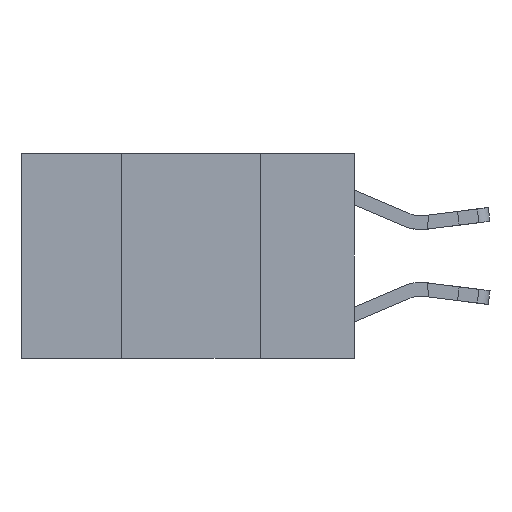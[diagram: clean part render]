
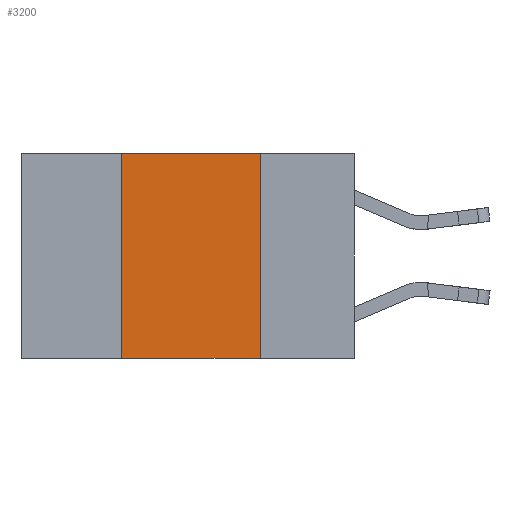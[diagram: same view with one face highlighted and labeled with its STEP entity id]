
A CAD part, left-side view. The second image highlights one B-rep face of the part: STEP entity #3200.
In plain terms, the highlighted planar face has unit normal (-1, 0, 0).
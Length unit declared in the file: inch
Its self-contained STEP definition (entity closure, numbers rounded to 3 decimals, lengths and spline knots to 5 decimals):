
#799 = VECTOR ( 'NONE', #19173, 39.37008 ) ;
#1078 = AXIS2_PLACEMENT_3D ( 'NONE', #11572, #17243, #7800 ) ;
#2281 = DIRECTION ( 'NONE',  ( 0., 0., -1. ) ) ;
#2421 = VERTEX_POINT ( 'NONE', #9214 ) ;
#2836 = VERTEX_POINT ( 'NONE', #13251 ) ;
#3200 = ADVANCED_FACE ( 'NONE', ( #12725 ), #14143, .F. ) ;
#3769 = LINE ( 'NONE', #14783, #11675 ) ;
#3931 = CARTESIAN_POINT ( 'NONE',  ( 0., 0.6, -0.37 ) ) ;
#4461 = LINE ( 'NONE', #11296, #799 ) ;
#6313 = ORIENTED_EDGE ( 'NONE', *, *, #10711, .F. ) ;
#7290 = ORIENTED_EDGE ( 'NONE', *, *, #11797, .T. ) ;
#7346 = VECTOR ( 'NONE', #13872, 39.37008 ) ;
#7543 = VERTEX_POINT ( 'NONE', #14776 ) ;
#7742 = VERTEX_POINT ( 'NONE', #16450 ) ;
#7800 = DIRECTION ( 'NONE',  ( 0., 0., -1. ) ) ;
#9214 = CARTESIAN_POINT ( 'NONE',  ( 0., 0.17, 0. ) ) ;
#10711 = EDGE_CURVE ( 'NONE', #7742, #7543, #15244, .T. ) ;
#11296 = CARTESIAN_POINT ( 'NONE',  ( 0., 0.6, 0. ) ) ;
#11572 = CARTESIAN_POINT ( 'NONE',  ( 0., 0.6, 0. ) ) ;
#11675 = VECTOR ( 'NONE', #2281, 39.37008 ) ;
#11797 = EDGE_CURVE ( 'NONE', #7742, #2836, #20089, .T. ) ;
#12265 = VECTOR ( 'NONE', #13404, 39.37008 ) ;
#12505 = EDGE_LOOP ( 'NONE', ( #15885, #12742, #6313, #7290 ) ) ;
#12725 = FACE_OUTER_BOUND ( 'NONE', #12505, .T. ) ;
#12742 = ORIENTED_EDGE ( 'NONE', *, *, #15253, .F. ) ;
#13251 = CARTESIAN_POINT ( 'NONE',  ( 0., 0.17, -0.37 ) ) ;
#13404 = DIRECTION ( 'NONE',  ( 0., -1., 0. ) ) ;
#13872 = DIRECTION ( 'NONE',  ( 0., 0., 1. ) ) ;
#13922 = EDGE_CURVE ( 'NONE', #2421, #2836, #3769, .T. ) ;
#14143 = PLANE ( 'NONE',  #1078 ) ;
#14776 = CARTESIAN_POINT ( 'NONE',  ( 0., 0.42, 0. ) ) ;
#14783 = CARTESIAN_POINT ( 'NONE',  ( 0., 0.17, 0. ) ) ;
#15244 = LINE ( 'NONE', #18577, #7346 ) ;
#15253 = EDGE_CURVE ( 'NONE', #7543, #2421, #4461, .T. ) ;
#15885 = ORIENTED_EDGE ( 'NONE', *, *, #13922, .F. ) ;
#16450 = CARTESIAN_POINT ( 'NONE',  ( 0., 0.42, -0.37 ) ) ;
#17243 = DIRECTION ( 'NONE',  ( 1., 0., 0. ) ) ;
#18577 = CARTESIAN_POINT ( 'NONE',  ( 0., 0.42, 0. ) ) ;
#19173 = DIRECTION ( 'NONE',  ( 0., -1., 0. ) ) ;
#20089 = LINE ( 'NONE', #3931, #12265 ) ;
